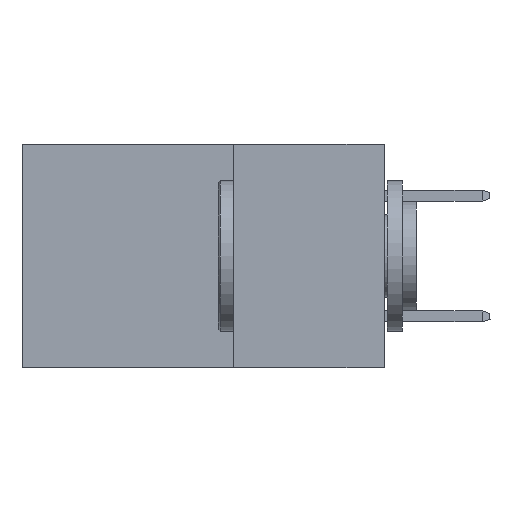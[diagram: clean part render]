
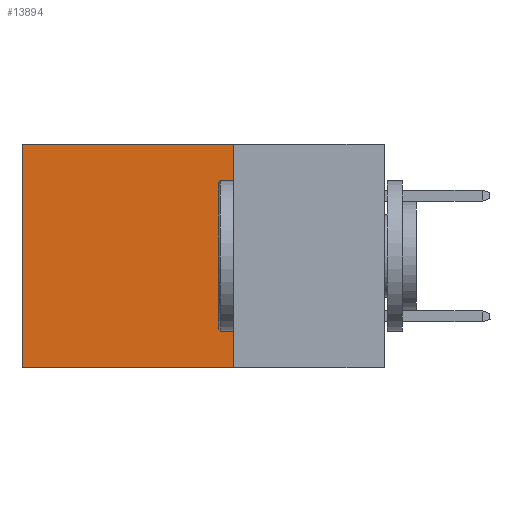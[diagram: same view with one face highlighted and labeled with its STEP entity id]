
A CAD part, left-side view. The second image highlights one B-rep face of the part: STEP entity #13894.
In plain terms, the highlighted planar face has unit normal (-1, 0, 0).
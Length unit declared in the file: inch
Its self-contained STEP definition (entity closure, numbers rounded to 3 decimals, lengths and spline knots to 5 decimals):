
#896 = CARTESIAN_POINT ( 'NONE',  ( 0.2615, 0.25, 0. ) ) ;
#1155 = CARTESIAN_POINT ( 'NONE',  ( 0.2615, 0.6, 0. ) ) ;
#2242 = CARTESIAN_POINT ( 'NONE',  ( 0.2615, 0.25, -0.37 ) ) ;
#2888 = ORIENTED_EDGE ( 'NONE', *, *, #16375, .F. ) ;
#3544 = VECTOR ( 'NONE', #16068, 39.37008 ) ;
#3713 = AXIS2_PLACEMENT_3D ( 'NONE', #2242, #13902, #3914 ) ;
#3914 = DIRECTION ( 'NONE',  ( 0., 0., -1. ) ) ;
#4696 = DIRECTION ( 'NONE',  ( 0., 0., -1. ) ) ;
#4759 = ORIENTED_EDGE ( 'NONE', *, *, #12970, .T. ) ;
#5166 = VERTEX_POINT ( 'NONE', #17904 ) ;
#5645 = ORIENTED_EDGE ( 'NONE', *, *, #11731, .T. ) ;
#6388 = VECTOR ( 'NONE', #16235, 39.37008 ) ;
#7906 = EDGE_LOOP ( 'NONE', ( #4759, #18663, #2888, #5645 ) ) ;
#8122 = LINE ( 'NONE', #12999, #12026 ) ;
#9479 = VECTOR ( 'NONE', #19677, 39.37008 ) ;
#9520 = CARTESIAN_POINT ( 'NONE',  ( 0.2615, 0.25, -0.37 ) ) ;
#10812 = FACE_OUTER_BOUND ( 'NONE', #7906, .T. ) ;
#11083 = EDGE_CURVE ( 'NONE', #5166, #15006, #19691, .T. ) ;
#11299 = CARTESIAN_POINT ( 'NONE',  ( 0.2615, 0.6, -0.37 ) ) ;
#11668 = CARTESIAN_POINT ( 'NONE',  ( 0.2615, 0.6, -0.37 ) ) ;
#11731 = EDGE_CURVE ( 'NONE', #18346, #19782, #12411, .T. ) ;
#12026 = VECTOR ( 'NONE', #4696, 39.37008 ) ;
#12232 = PLANE ( 'NONE',  #3713 ) ;
#12411 = LINE ( 'NONE', #14368, #3544 ) ;
#12970 = EDGE_CURVE ( 'NONE', #19782, #15006, #18884, .T. ) ;
#12999 = CARTESIAN_POINT ( 'NONE',  ( 0.2615, 0.25, -0.37 ) ) ;
#13894 = ADVANCED_FACE ( 'NONE', ( #10812 ), #12232, .F. ) ;
#13902 = DIRECTION ( 'NONE',  ( 1., 0., 0. ) ) ;
#14368 = CARTESIAN_POINT ( 'NONE',  ( 0.2615, 0.25, 0. ) ) ;
#15006 = VERTEX_POINT ( 'NONE', #11668 ) ;
#16068 = DIRECTION ( 'NONE',  ( 0., 1., 0. ) ) ;
#16235 = DIRECTION ( 'NONE',  ( 0., 1., 0. ) ) ;
#16375 = EDGE_CURVE ( 'NONE', #18346, #5166, #8122, .T. ) ;
#17904 = CARTESIAN_POINT ( 'NONE',  ( 0.2615, 0.25, -0.37 ) ) ;
#18346 = VERTEX_POINT ( 'NONE', #896 ) ;
#18663 = ORIENTED_EDGE ( 'NONE', *, *, #11083, .F. ) ;
#18884 = LINE ( 'NONE', #11299, #9479 ) ;
#19677 = DIRECTION ( 'NONE',  ( 0., 0., -1. ) ) ;
#19691 = LINE ( 'NONE', #9520, #6388 ) ;
#19782 = VERTEX_POINT ( 'NONE', #1155 ) ;
